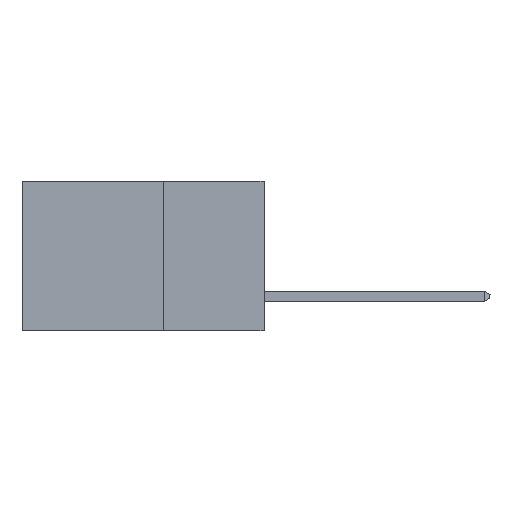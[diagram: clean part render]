
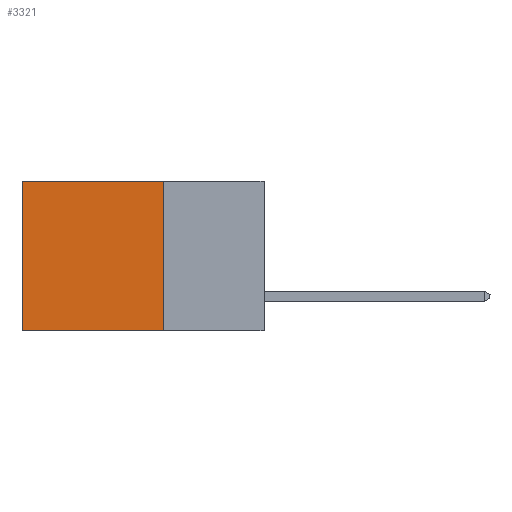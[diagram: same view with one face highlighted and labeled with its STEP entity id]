
A CAD part, left-side view. The second image highlights one B-rep face of the part: STEP entity #3321.
In plain terms, the highlighted planar face has unit normal (-1, 0, 0).
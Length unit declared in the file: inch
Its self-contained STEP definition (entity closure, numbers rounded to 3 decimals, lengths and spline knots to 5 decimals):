
#551 = ORIENTED_EDGE ( 'NONE', *, *, #4371, .F. ) ;
#820 = VECTOR ( 'NONE', #8294, 39.37008 ) ;
#962 = VECTOR ( 'NONE', #5900, 39.37008 ) ;
#1008 = DIRECTION ( 'NONE',  ( 0., 1., 0. ) ) ;
#1474 = ORIENTED_EDGE ( 'NONE', *, *, #8034, .T. ) ;
#1878 = DIRECTION ( 'NONE',  ( 0., 0., -1. ) ) ;
#2026 = VECTOR ( 'NONE', #1878, 39.37008 ) ;
#2572 = DIRECTION ( 'NONE',  ( 1., 0., 0. ) ) ;
#3321 = ADVANCED_FACE ( 'NONE', ( #9002 ), #7501, .F. ) ;
#3742 = CARTESIAN_POINT ( 'NONE',  ( 0.2615, 0.6, -0.37 ) ) ;
#3768 = CARTESIAN_POINT ( 'NONE',  ( 0.2615, 0.25, 0. ) ) ;
#3827 = VERTEX_POINT ( 'NONE', #3768 ) ;
#4371 = EDGE_CURVE ( 'NONE', #9155, #9461, #9342, .T. ) ;
#4729 = CARTESIAN_POINT ( 'NONE',  ( 0.2615, 0.25, -0.37 ) ) ;
#4836 = DIRECTION ( 'NONE',  ( 0., 0., -1. ) ) ;
#4963 = LINE ( 'NONE', #8589, #7577 ) ;
#4971 = ORIENTED_EDGE ( 'NONE', *, *, #10045, .F. ) ;
#5844 = AXIS2_PLACEMENT_3D ( 'NONE', #9056, #2572, #4836 ) ;
#5900 = DIRECTION ( 'NONE',  ( 0., 1., 0. ) ) ;
#6059 = CARTESIAN_POINT ( 'NONE',  ( 0.2615, 0.6, -0.37 ) ) ;
#6651 = LINE ( 'NONE', #4729, #820 ) ;
#7501 = PLANE ( 'NONE',  #5844 ) ;
#7577 = VECTOR ( 'NONE', #1008, 39.37008 ) ;
#7973 = EDGE_CURVE ( 'NONE', #3827, #10183, #4963, .T. ) ;
#8034 = EDGE_CURVE ( 'NONE', #10183, #9461, #9339, .T. ) ;
#8294 = DIRECTION ( 'NONE',  ( 0., 0., -1. ) ) ;
#8538 = CARTESIAN_POINT ( 'NONE',  ( 0.2615, 0.25, -0.37 ) ) ;
#8589 = CARTESIAN_POINT ( 'NONE',  ( 0.2615, 0.25, 0. ) ) ;
#8668 = ORIENTED_EDGE ( 'NONE', *, *, #7973, .T. ) ;
#9002 = FACE_OUTER_BOUND ( 'NONE', #9808, .T. ) ;
#9056 = CARTESIAN_POINT ( 'NONE',  ( 0.2615, 0.25, -0.37 ) ) ;
#9155 = VERTEX_POINT ( 'NONE', #9837 ) ;
#9272 = CARTESIAN_POINT ( 'NONE',  ( 0.2615, 0.6, 0. ) ) ;
#9339 = LINE ( 'NONE', #6059, #2026 ) ;
#9342 = LINE ( 'NONE', #8538, #962 ) ;
#9461 = VERTEX_POINT ( 'NONE', #3742 ) ;
#9808 = EDGE_LOOP ( 'NONE', ( #1474, #551, #4971, #8668 ) ) ;
#9837 = CARTESIAN_POINT ( 'NONE',  ( 0.2615, 0.25, -0.37 ) ) ;
#10045 = EDGE_CURVE ( 'NONE', #3827, #9155, #6651, .T. ) ;
#10183 = VERTEX_POINT ( 'NONE', #9272 ) ;
